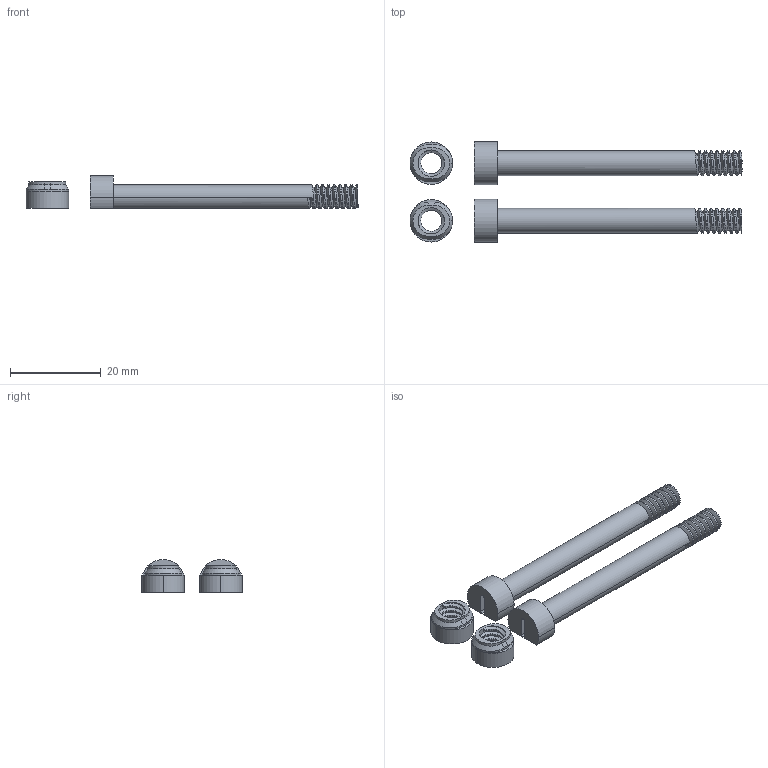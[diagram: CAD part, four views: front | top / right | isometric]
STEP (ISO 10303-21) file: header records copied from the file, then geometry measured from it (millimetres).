
FILE_DESCRIPTION (( 'STEP AP203' ), '1' );
FILE_NAME ('AF-WF-VF-MDL-001-STEP.STEP', '2020-07-22T01:06:39', ( '' ), ( '' ), 'SwSTEP 2.0', 'SolidWorks 2018', '' );
FILE_SCHEMA (( 'CONFIG_CONTROL_DESIGN' ));
Length unit declared in the file: inch
Products named in the file (1): AF-WF-VF-MDL-001-STEP
Bounding box: 73.28 x 22.23 x 7.24 mm (x, y, z)
Volume: 3423.5 mm3; surface area: 3363.9 mm2
Topology: 4 solids, 4 shells, 176 faces, 466 edges, 298 vertices
Faces by surface type: cylinder 104, plane 54, bspline 12, cone 6
Entity records: 9533 total; most frequent: CARTESIAN_POINT 5615, ORIENTED_EDGE 932, DIRECTION 678, EDGE_CURVE 466, VERTEX_POINT 298, AXIS2_PLACEMENT_3D 241, LINE 196, VECTOR 196
